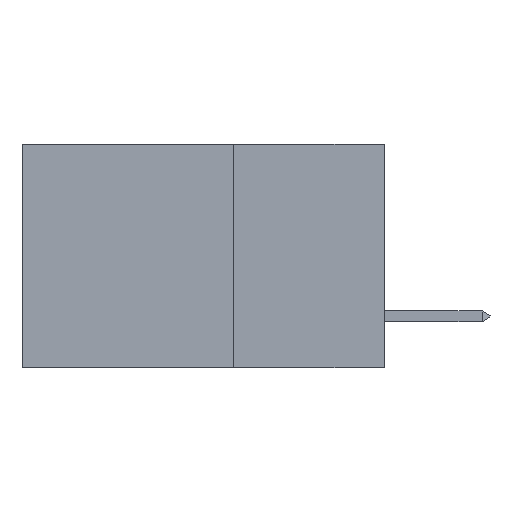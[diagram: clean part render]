
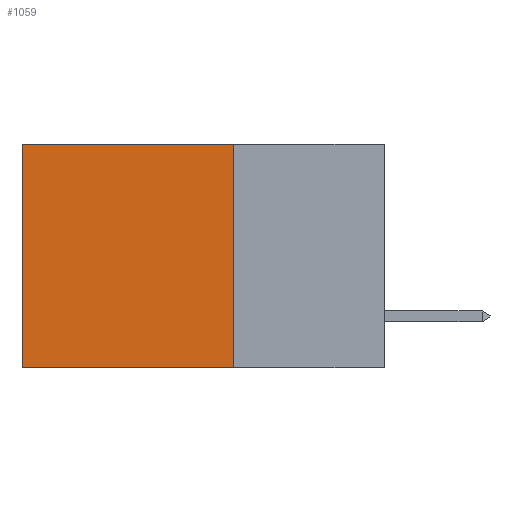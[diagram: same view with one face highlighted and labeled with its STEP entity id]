
A CAD part, left-side view. The second image highlights one B-rep face of the part: STEP entity #1059.
In plain terms, the highlighted planar face has unit normal (-1, 0, 0).
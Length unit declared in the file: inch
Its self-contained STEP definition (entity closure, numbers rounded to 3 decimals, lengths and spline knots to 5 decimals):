
#599 = CARTESIAN_POINT ( 'NONE',  ( 0.2875, 0.6, 0. ) ) ;
#794 = ORIENTED_EDGE ( 'NONE', *, *, #3731, .T. ) ;
#1059 = ADVANCED_FACE ( 'NONE', ( #18640 ), #14726, .F. ) ;
#3728 = CARTESIAN_POINT ( 'NONE',  ( 0.2875, 0.25, -0.37 ) ) ;
#3731 = EDGE_CURVE ( 'NONE', #9470, #8174, #21671, .T. ) ;
#3908 = CARTESIAN_POINT ( 'NONE',  ( 0.2875, 0.25, 0. ) ) ;
#3912 = CARTESIAN_POINT ( 'NONE',  ( 0.2875, 0.25, 0. ) ) ;
#4081 = EDGE_CURVE ( 'NONE', #20915, #6694, #12266, .T. ) ;
#4888 = ORIENTED_EDGE ( 'NONE', *, *, #4081, .F. ) ;
#6694 = VERTEX_POINT ( 'NONE', #7258 ) ;
#6706 = EDGE_CURVE ( 'NONE', #9470, #20915, #20195, .T. ) ;
#6722 = CARTESIAN_POINT ( 'NONE',  ( 0.2875, 0.6, 0. ) ) ;
#6869 = EDGE_LOOP ( 'NONE', ( #18931, #4888, #11801, #794 ) ) ;
#7258 = CARTESIAN_POINT ( 'NONE',  ( 0.2875, 0.6, -0.37 ) ) ;
#7718 = DIRECTION ( 'NONE',  ( 0., 0., -1. ) ) ;
#8174 = VERTEX_POINT ( 'NONE', #599 ) ;
#9144 = DIRECTION ( 'NONE',  ( 1., 0., 0. ) ) ;
#9470 = VERTEX_POINT ( 'NONE', #20115 ) ;
#10046 = LINE ( 'NONE', #6722, #10080 ) ;
#10080 = VECTOR ( 'NONE', #11828, 39.37008 ) ;
#11797 = CARTESIAN_POINT ( 'NONE',  ( 0.2875, 0.25, -0.37 ) ) ;
#11801 = ORIENTED_EDGE ( 'NONE', *, *, #6706, .F. ) ;
#11828 = DIRECTION ( 'NONE',  ( 0., 0., -1. ) ) ;
#12266 = LINE ( 'NONE', #11797, #23185 ) ;
#14726 = PLANE ( 'NONE',  #22573 ) ;
#16179 = DIRECTION ( 'NONE',  ( 0., 0., -1. ) ) ;
#16318 = DIRECTION ( 'NONE',  ( 0., 1., 0. ) ) ;
#16434 = CARTESIAN_POINT ( 'NONE',  ( 0.2875, 0.25, 0. ) ) ;
#18640 = FACE_OUTER_BOUND ( 'NONE', #6869, .T. ) ;
#18931 = ORIENTED_EDGE ( 'NONE', *, *, #19386, .T. ) ;
#19386 = EDGE_CURVE ( 'NONE', #8174, #6694, #10046, .T. ) ;
#20115 = CARTESIAN_POINT ( 'NONE',  ( 0.2875, 0.25, 0. ) ) ;
#20195 = LINE ( 'NONE', #3912, #21765 ) ;
#20915 = VERTEX_POINT ( 'NONE', #3728 ) ;
#21069 = DIRECTION ( 'NONE',  ( 0., 1., 0. ) ) ;
#21671 = LINE ( 'NONE', #16434, #21714 ) ;
#21714 = VECTOR ( 'NONE', #16318, 39.37008 ) ;
#21765 = VECTOR ( 'NONE', #16179, 39.37008 ) ;
#22573 = AXIS2_PLACEMENT_3D ( 'NONE', #3908, #9144, #7718 ) ;
#23185 = VECTOR ( 'NONE', #21069, 39.37008 ) ;
